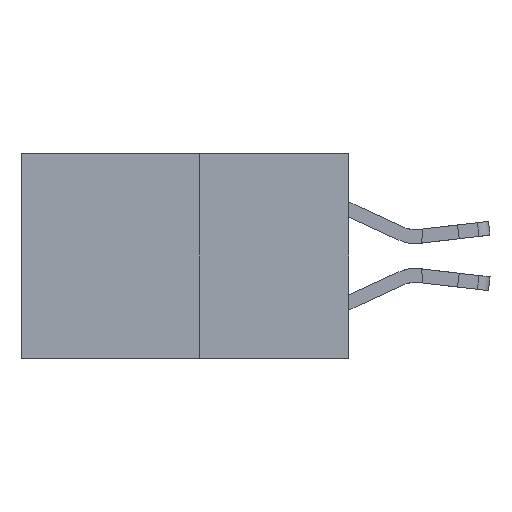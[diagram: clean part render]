
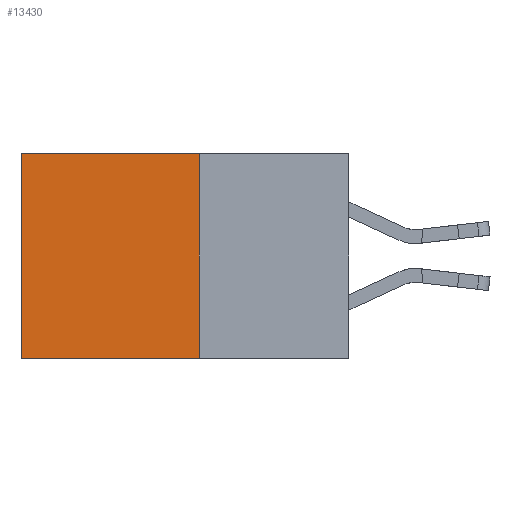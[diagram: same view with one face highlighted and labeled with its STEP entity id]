
A CAD part, left-side view. The second image highlights one B-rep face of the part: STEP entity #13430.
In plain terms, the highlighted planar face has unit normal (-1, 0, 0).
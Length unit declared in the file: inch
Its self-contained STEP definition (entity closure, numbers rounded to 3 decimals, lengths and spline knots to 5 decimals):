
#411 = PLANE ( 'NONE',  #6686 ) ;
#1873 = ORIENTED_EDGE ( 'NONE', *, *, #9448, .T. ) ;
#1948 = VECTOR ( 'NONE', #5937, 39.37008 ) ;
#2729 = VERTEX_POINT ( 'NONE', #10219 ) ;
#2758 = CARTESIAN_POINT ( 'NONE',  ( 0.277, 0.27, -0.37 ) ) ;
#3437 = ORIENTED_EDGE ( 'NONE', *, *, #13227, .T. ) ;
#3567 = ORIENTED_EDGE ( 'NONE', *, *, #5793, .F. ) ;
#3590 = CARTESIAN_POINT ( 'NONE',  ( 0.277, 0.27, 0. ) ) ;
#3933 = DIRECTION ( 'NONE',  ( 0., 0., -1. ) ) ;
#4619 = CARTESIAN_POINT ( 'NONE',  ( 0.277, 0.59, -0.37 ) ) ;
#5408 = LINE ( 'NONE', #4619, #14291 ) ;
#5793 = EDGE_CURVE ( 'NONE', #2729, #12295, #7578, .T. ) ;
#5842 = DIRECTION ( 'NONE',  ( 0., 0., -1. ) ) ;
#5937 = DIRECTION ( 'NONE',  ( 0., 1., 0. ) ) ;
#6686 = AXIS2_PLACEMENT_3D ( 'NONE', #2758, #10979, #3933 ) ;
#6765 = DIRECTION ( 'NONE',  ( 0., 0., -1. ) ) ;
#6826 = VECTOR ( 'NONE', #10872, 39.37008 ) ;
#7090 = VECTOR ( 'NONE', #6765, 39.37008 ) ;
#7544 = LINE ( 'NONE', #12880, #1948 ) ;
#7578 = LINE ( 'NONE', #9714, #6826 ) ;
#7704 = FACE_OUTER_BOUND ( 'NONE', #10759, .T. ) ;
#9448 = EDGE_CURVE ( 'NONE', #13155, #12295, #5408, .T. ) ;
#9714 = CARTESIAN_POINT ( 'NONE',  ( 0.277, 0.27, -0.37 ) ) ;
#9982 = EDGE_CURVE ( 'NONE', #10208, #2729, #10545, .T. ) ;
#10208 = VERTEX_POINT ( 'NONE', #3590 ) ;
#10219 = CARTESIAN_POINT ( 'NONE',  ( 0.277, 0.27, -0.37 ) ) ;
#10545 = LINE ( 'NONE', #11440, #7090 ) ;
#10759 = EDGE_LOOP ( 'NONE', ( #1873, #3567, #13278, #3437 ) ) ;
#10872 = DIRECTION ( 'NONE',  ( 0., 1., 0. ) ) ;
#10979 = DIRECTION ( 'NONE',  ( 1., 0., 0. ) ) ;
#11264 = CARTESIAN_POINT ( 'NONE',  ( 0.277, 0.59, -0.37 ) ) ;
#11440 = CARTESIAN_POINT ( 'NONE',  ( 0.277, 0.27, -0.37 ) ) ;
#12295 = VERTEX_POINT ( 'NONE', #11264 ) ;
#12880 = CARTESIAN_POINT ( 'NONE',  ( 0.277, 0.27, 0. ) ) ;
#13155 = VERTEX_POINT ( 'NONE', #13826 ) ;
#13227 = EDGE_CURVE ( 'NONE', #10208, #13155, #7544, .T. ) ;
#13278 = ORIENTED_EDGE ( 'NONE', *, *, #9982, .F. ) ;
#13430 = ADVANCED_FACE ( 'NONE', ( #7704 ), #411, .F. ) ;
#13826 = CARTESIAN_POINT ( 'NONE',  ( 0.277, 0.59, 0. ) ) ;
#14291 = VECTOR ( 'NONE', #5842, 39.37008 ) ;
